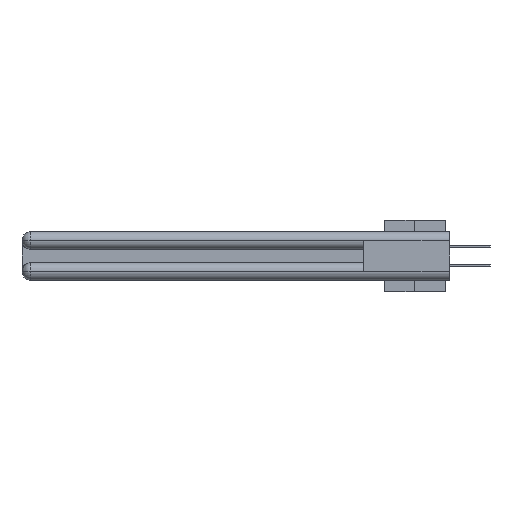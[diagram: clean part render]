
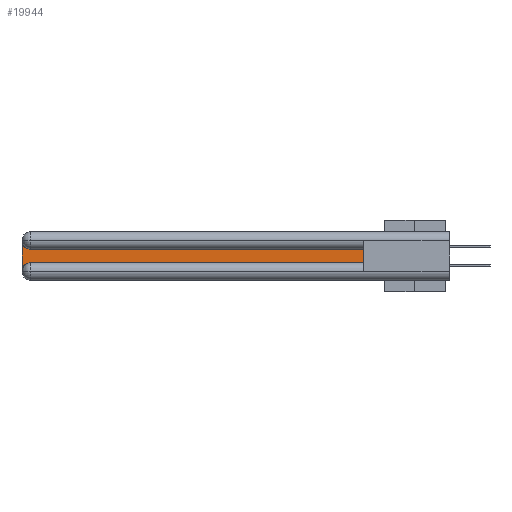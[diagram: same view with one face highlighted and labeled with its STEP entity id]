
A CAD part, left-side view. The second image highlights one B-rep face of the part: STEP entity #19944.
In plain terms, the highlighted planar face has unit normal (-1, 0, 0).
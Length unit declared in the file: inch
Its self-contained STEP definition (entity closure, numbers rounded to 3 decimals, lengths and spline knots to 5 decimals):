
#18 = DIRECTION ( 'NONE',  ( 0., 0., -1. ) ) ;
#1281 = CARTESIAN_POINT ( 'NONE',  ( 0.075, 3., -0.1225 ) ) ;
#2219 = ORIENTED_EDGE ( 'NONE', *, *, #38094, .T. ) ;
#4750 = VERTEX_POINT ( 'NONE', #38284 ) ;
#4998 = DIRECTION ( 'NONE',  ( 0., 0., -1. ) ) ;
#5984 = ORIENTED_EDGE ( 'NONE', *, *, #36743, .T. ) ;
#6268 = EDGE_CURVE ( 'NONE', #7437, #12121, #6540, .T. ) ;
#6540 = LINE ( 'NONE', #26834, #31047 ) ;
#6838 = AXIS2_PLACEMENT_3D ( 'NONE', #6881, #19135, #18 ) ;
#6881 = CARTESIAN_POINT ( 'NONE',  ( 0.075, 2.94, -0.0625 ) ) ;
#7437 = VERTEX_POINT ( 'NONE', #23748 ) ;
#7847 = CARTESIAN_POINT ( 'NONE',  ( 0.075, 2.94, -0.2775 ) ) ;
#8583 = DIRECTION ( 'NONE',  ( 0., 1., 0. ) ) ;
#9829 = LINE ( 'NONE', #24216, #20834 ) ;
#10955 = CARTESIAN_POINT ( 'NONE',  ( 0.075, 0.6, -0.1225 ) ) ;
#12121 = VERTEX_POINT ( 'NONE', #10955 ) ;
#13374 = DIRECTION ( 'NONE',  ( 0., 0., 1. ) ) ;
#14225 = DIRECTION ( 'NONE',  ( 1., 0., 0. ) ) ;
#14495 = ORIENTED_EDGE ( 'NONE', *, *, #6268, .T. ) ;
#14830 = VERTEX_POINT ( 'NONE', #37497 ) ;
#14953 = VECTOR ( 'NONE', #8583, 39.37008 ) ;
#16263 = VECTOR ( 'NONE', #27784, 39.37008 ) ;
#19135 = DIRECTION ( 'NONE',  ( 1., 0., 0. ) ) ;
#19500 = LINE ( 'NONE', #37380, #14953 ) ;
#19944 = ADVANCED_FACE ( 'NONE', ( #22158 ), #39011, .F. ) ;
#20247 = AXIS2_PLACEMENT_3D ( 'NONE', #1281, #30201, #33242 ) ;
#20834 = VECTOR ( 'NONE', #4998, 39.37008 ) ;
#22073 = CIRCLE ( 'NONE', #34429, 0.06 ) ;
#22158 = FACE_OUTER_BOUND ( 'NONE', #25991, .T. ) ;
#23748 = CARTESIAN_POINT ( 'NONE',  ( 0.075, 0.6, -0.2175 ) ) ;
#24216 = CARTESIAN_POINT ( 'NONE',  ( 0.075, 3., -0.2175 ) ) ;
#25991 = EDGE_LOOP ( 'NONE', ( #40652, #40460, #5984, #28467, #2219, #14495 ) ) ;
#26834 = CARTESIAN_POINT ( 'NONE',  ( 0.075, 0.6, -0.2175 ) ) ;
#27784 = DIRECTION ( 'NONE',  ( 0., -1., 0. ) ) ;
#27856 = DIRECTION ( 'NONE',  ( 0., 0., -1. ) ) ;
#28467 = ORIENTED_EDGE ( 'NONE', *, *, #39216, .T. ) ;
#28469 = VERTEX_POINT ( 'NONE', #37284 ) ;
#30201 = DIRECTION ( 'NONE',  ( 1., 0., 0. ) ) ;
#30718 = CARTESIAN_POINT ( 'NONE',  ( 0.075, 2.94, -0.2175 ) ) ;
#31047 = VECTOR ( 'NONE', #13374, 39.37008 ) ;
#33242 = DIRECTION ( 'NONE',  ( 0., 0., -1. ) ) ;
#34429 = AXIS2_PLACEMENT_3D ( 'NONE', #7847, #14225, #27856 ) ;
#35300 = LINE ( 'NONE', #36168, #16263 ) ;
#36168 = CARTESIAN_POINT ( 'NONE',  ( 0.075, 0.6, -0.2175 ) ) ;
#36743 = EDGE_CURVE ( 'NONE', #14830, #28469, #9829, .T. ) ;
#37284 = CARTESIAN_POINT ( 'NONE',  ( 0.075, 3., -0.2775 ) ) ;
#37380 = CARTESIAN_POINT ( 'NONE',  ( 0.075, 0.6, -0.1225 ) ) ;
#37497 = CARTESIAN_POINT ( 'NONE',  ( 0.075, 3., -0.0625 ) ) ;
#38094 = EDGE_CURVE ( 'NONE', #38103, #7437, #35300, .T. ) ;
#38103 = VERTEX_POINT ( 'NONE', #30718 ) ;
#38284 = CARTESIAN_POINT ( 'NONE',  ( 0.075, 2.94, -0.1225 ) ) ;
#38457 = EDGE_CURVE ( 'NONE', #4750, #14830, #40242, .T. ) ;
#39011 = PLANE ( 'NONE',  #20247 ) ;
#39216 = EDGE_CURVE ( 'NONE', #28469, #38103, #22073, .T. ) ;
#39978 = EDGE_CURVE ( 'NONE', #12121, #4750, #19500, .T. ) ;
#40242 = CIRCLE ( 'NONE', #6838, 0.06 ) ;
#40460 = ORIENTED_EDGE ( 'NONE', *, *, #38457, .T. ) ;
#40652 = ORIENTED_EDGE ( 'NONE', *, *, #39978, .T. ) ;
